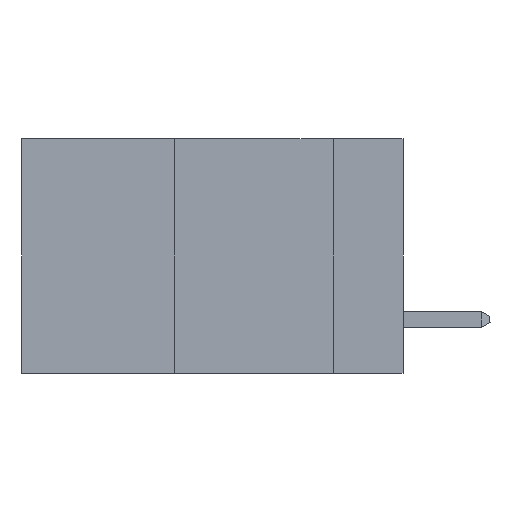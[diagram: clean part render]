
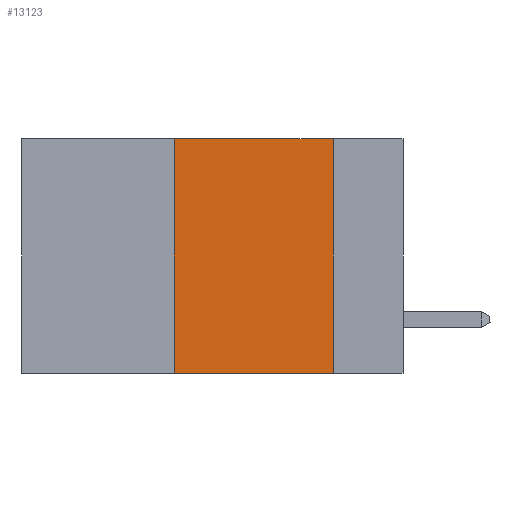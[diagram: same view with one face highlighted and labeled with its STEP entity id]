
A CAD part, left-side view. The second image highlights one B-rep face of the part: STEP entity #13123.
In plain terms, the highlighted planar face has unit normal (-1, 0, 0).
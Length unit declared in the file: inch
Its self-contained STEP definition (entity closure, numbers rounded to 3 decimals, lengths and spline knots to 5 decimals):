
#528 = LINE ( 'NONE', #41031, #40967 ) ;
#1159 = ORIENTED_EDGE ( 'NONE', *, *, #9480, .F. ) ;
#1192 = CARTESIAN_POINT ( 'NONE',  ( 0., 0.6, 0. ) ) ;
#1623 = EDGE_CURVE ( 'NONE', #22219, #3568, #41809, .T. ) ;
#2416 = CARTESIAN_POINT ( 'NONE',  ( 0., 0.36, 0. ) ) ;
#3093 = DIRECTION ( 'NONE',  ( 0., 0., -1. ) ) ;
#3494 = AXIS2_PLACEMENT_3D ( 'NONE', #9887, #39383, #43072 ) ;
#3568 = VERTEX_POINT ( 'NONE', #28821 ) ;
#3804 = LINE ( 'NONE', #1192, #4357 ) ;
#4357 = VECTOR ( 'NONE', #42823, 39.37008 ) ;
#9176 = CARTESIAN_POINT ( 'NONE',  ( 0., 0.36, 0. ) ) ;
#9480 = EDGE_CURVE ( 'NONE', #14074, #37528, #3804, .T. ) ;
#9530 = CARTESIAN_POINT ( 'NONE',  ( 0., 0.36, -0.37 ) ) ;
#9887 = CARTESIAN_POINT ( 'NONE',  ( 0., 0.6, 0. ) ) ;
#9979 = LINE ( 'NONE', #2416, #11662 ) ;
#10062 = CARTESIAN_POINT ( 'NONE',  ( 0., 0.6, -0.37 ) ) ;
#11662 = VECTOR ( 'NONE', #31954, 39.37008 ) ;
#12603 = FACE_OUTER_BOUND ( 'NONE', #13960, .T. ) ;
#12958 = EDGE_CURVE ( 'NONE', #37528, #3568, #528, .T. ) ;
#13123 = ADVANCED_FACE ( 'NONE', ( #12603 ), #40021, .F. ) ;
#13960 = EDGE_LOOP ( 'NONE', ( #44919, #1159, #21149, #15243 ) ) ;
#14074 = VERTEX_POINT ( 'NONE', #9176 ) ;
#15243 = ORIENTED_EDGE ( 'NONE', *, *, #1623, .T. ) ;
#21149 = ORIENTED_EDGE ( 'NONE', *, *, #37717, .F. ) ;
#22219 = VERTEX_POINT ( 'NONE', #9530 ) ;
#28821 = CARTESIAN_POINT ( 'NONE',  ( 0., 0.11, -0.37 ) ) ;
#31812 = DIRECTION ( 'NONE',  ( 0., -1., 0. ) ) ;
#31954 = DIRECTION ( 'NONE',  ( 0., 0., 1. ) ) ;
#37528 = VERTEX_POINT ( 'NONE', #44595 ) ;
#37717 = EDGE_CURVE ( 'NONE', #22219, #14074, #9979, .T. ) ;
#38345 = VECTOR ( 'NONE', #31812, 39.37008 ) ;
#39383 = DIRECTION ( 'NONE',  ( 1., 0., 0. ) ) ;
#40021 = PLANE ( 'NONE',  #3494 ) ;
#40967 = VECTOR ( 'NONE', #3093, 39.37008 ) ;
#41031 = CARTESIAN_POINT ( 'NONE',  ( 0., 0.11, 0. ) ) ;
#41809 = LINE ( 'NONE', #10062, #38345 ) ;
#42823 = DIRECTION ( 'NONE',  ( 0., -1., 0. ) ) ;
#43072 = DIRECTION ( 'NONE',  ( 0., 0., -1. ) ) ;
#44595 = CARTESIAN_POINT ( 'NONE',  ( 0., 0.11, 0. ) ) ;
#44919 = ORIENTED_EDGE ( 'NONE', *, *, #12958, .F. ) ;
